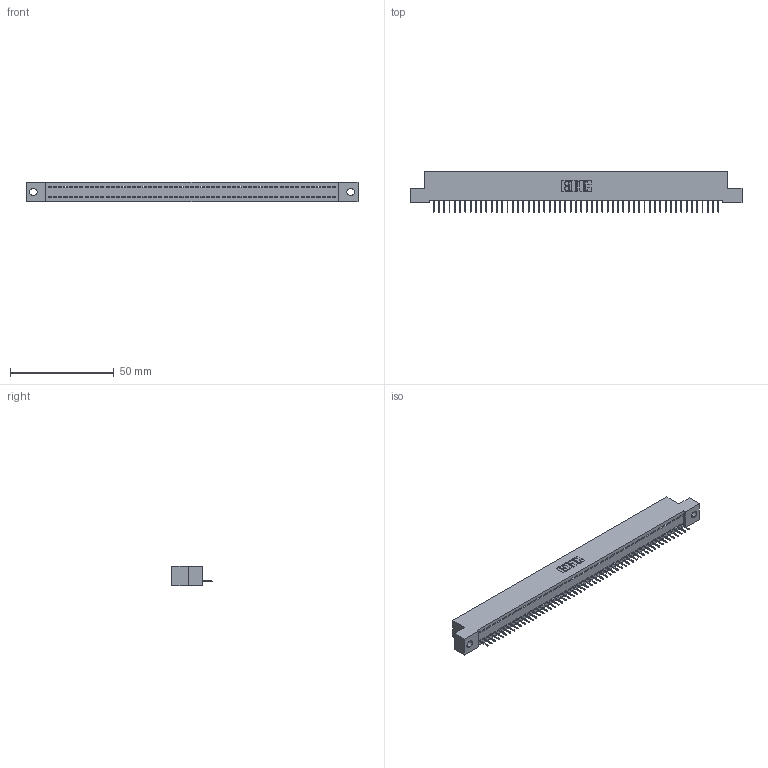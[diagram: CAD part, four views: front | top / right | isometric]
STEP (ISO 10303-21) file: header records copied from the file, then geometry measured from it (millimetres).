
FILE_DESCRIPTION (( 'STEP AP203' ), '1' );
FILE_NAME ('342-055-524-102.STEP', '2019-10-03T04:03:09', ( '' ), ( '' ), 'SwSTEP 2.0', 'SolidWorks 2016', '' );
FILE_SCHEMA (( 'CONFIG_CONTROL_DESIGN' ));
Length unit declared in the file: inch
Products named in the file (3): 342-055-524-102; 342 Part_.128 Slot; 345-292-001_345-293-124
Assembly tree (56 placements, depth 2):
  342-055-524-102
    342 Part_.128 Slot
    345-292-001_345-293-124  x55
Bounding box: 160.02 x 19.69 x 9.4 mm (x, y, z)
Volume: 13809 mm3; surface area: 19605.4 mm2
Topology: 56 solids, 56 shells, 3524 faces, 10211 edges, 6586 vertices
Faces by surface type: plane 2710, cylinder 814
Entity records: 32019 total; most frequent: CARTESIAN_POINT 5527, ORIENTED_EDGE 5518, DIRECTION 4637, EDGE_CURVE 2759, LINE 2635, VECTOR 2635, VERTEX_POINT 1834, AXIS2_PLACEMENT_3D 1001
